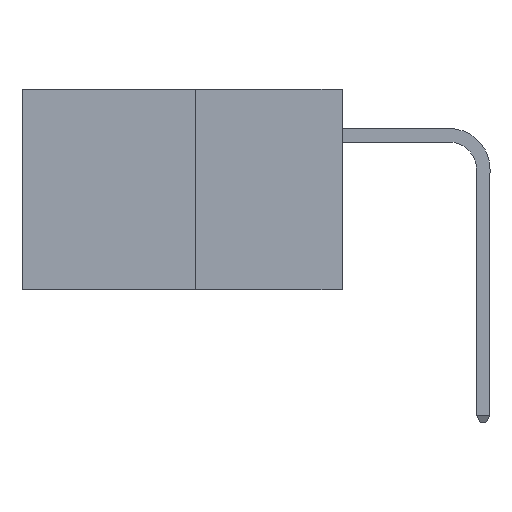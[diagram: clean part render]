
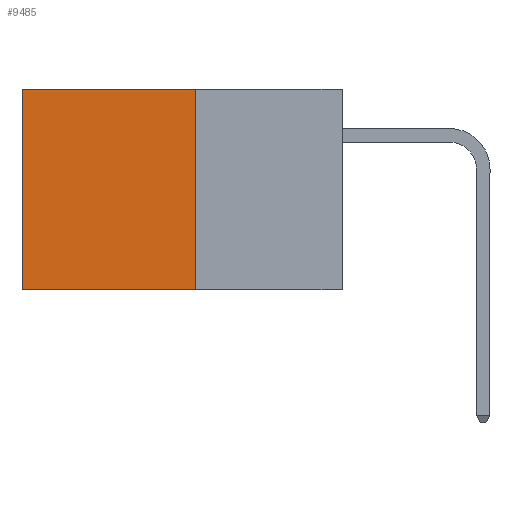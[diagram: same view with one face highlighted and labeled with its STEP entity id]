
A CAD part, left-side view. The second image highlights one B-rep face of the part: STEP entity #9485.
In plain terms, the highlighted planar face has unit normal (-1, 0, 0).
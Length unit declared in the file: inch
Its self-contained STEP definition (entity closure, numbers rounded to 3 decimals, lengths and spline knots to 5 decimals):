
#121 = CARTESIAN_POINT ( 'NONE',  ( 0.277, 0.27, -0.37 ) ) ;
#799 = ORIENTED_EDGE ( 'NONE', *, *, #6184, .F. ) ;
#940 = EDGE_CURVE ( 'NONE', #4300, #3375, #8169, .T. ) ;
#965 = LINE ( 'NONE', #121, #5283 ) ;
#1665 = EDGE_CURVE ( 'NONE', #1666, #3375, #6428, .T. ) ;
#1666 = VERTEX_POINT ( 'NONE', #4311 ) ;
#1988 = AXIS2_PLACEMENT_3D ( 'NONE', #5159, #5147, #5130 ) ;
#2287 = CARTESIAN_POINT ( 'NONE',  ( 0.277, 0.27, -0.37 ) ) ;
#2683 = VERTEX_POINT ( 'NONE', #7043 ) ;
#3375 = VERTEX_POINT ( 'NONE', #7534 ) ;
#3399 = DIRECTION ( 'NONE',  ( 0., 1., 0. ) ) ;
#3584 = CARTESIAN_POINT ( 'NONE',  ( 0.277, 0.27, 0. ) ) ;
#3786 = ORIENTED_EDGE ( 'NONE', *, *, #9752, .T. ) ;
#3927 = VECTOR ( 'NONE', #5216, 39.37008 ) ;
#4186 = DIRECTION ( 'NONE',  ( 0., 0., -1. ) ) ;
#4300 = VERTEX_POINT ( 'NONE', #2287 ) ;
#4311 = CARTESIAN_POINT ( 'NONE',  ( 0.277, 0.59, 0. ) ) ;
#4330 = CARTESIAN_POINT ( 'NONE',  ( 0.277, 0.59, -0.37 ) ) ;
#4437 = LINE ( 'NONE', #3584, #8424 ) ;
#4977 = CARTESIAN_POINT ( 'NONE',  ( 0.277, 0.27, -0.37 ) ) ;
#5130 = DIRECTION ( 'NONE',  ( 0., 0., -1. ) ) ;
#5147 = DIRECTION ( 'NONE',  ( 1., 0., 0. ) ) ;
#5159 = CARTESIAN_POINT ( 'NONE',  ( 0.277, 0.27, -0.37 ) ) ;
#5170 = PLANE ( 'NONE',  #1988 ) ;
#5216 = DIRECTION ( 'NONE',  ( 0., 1., 0. ) ) ;
#5283 = VECTOR ( 'NONE', #7645, 39.37008 ) ;
#6001 = EDGE_LOOP ( 'NONE', ( #6215, #8218, #799, #3786 ) ) ;
#6184 = EDGE_CURVE ( 'NONE', #2683, #4300, #965, .T. ) ;
#6215 = ORIENTED_EDGE ( 'NONE', *, *, #1665, .T. ) ;
#6428 = LINE ( 'NONE', #4330, #10086 ) ;
#7043 = CARTESIAN_POINT ( 'NONE',  ( 0.277, 0.27, 0. ) ) ;
#7192 = FACE_OUTER_BOUND ( 'NONE', #6001, .T. ) ;
#7534 = CARTESIAN_POINT ( 'NONE',  ( 0.277, 0.59, -0.37 ) ) ;
#7645 = DIRECTION ( 'NONE',  ( 0., 0., -1. ) ) ;
#8169 = LINE ( 'NONE', #4977, #3927 ) ;
#8218 = ORIENTED_EDGE ( 'NONE', *, *, #940, .F. ) ;
#8424 = VECTOR ( 'NONE', #3399, 39.37008 ) ;
#9485 = ADVANCED_FACE ( 'NONE', ( #7192 ), #5170, .F. ) ;
#9752 = EDGE_CURVE ( 'NONE', #2683, #1666, #4437, .T. ) ;
#10086 = VECTOR ( 'NONE', #4186, 39.37008 ) ;
